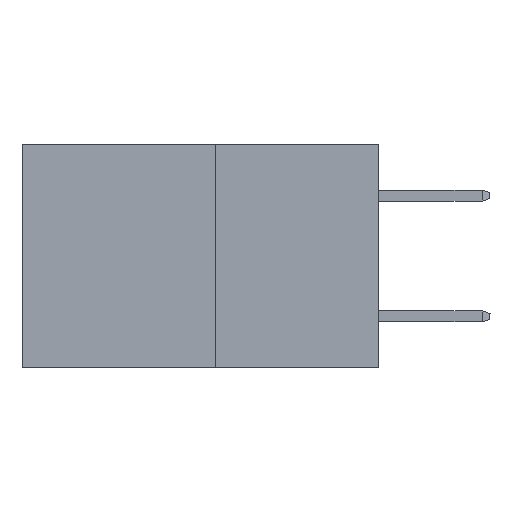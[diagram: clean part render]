
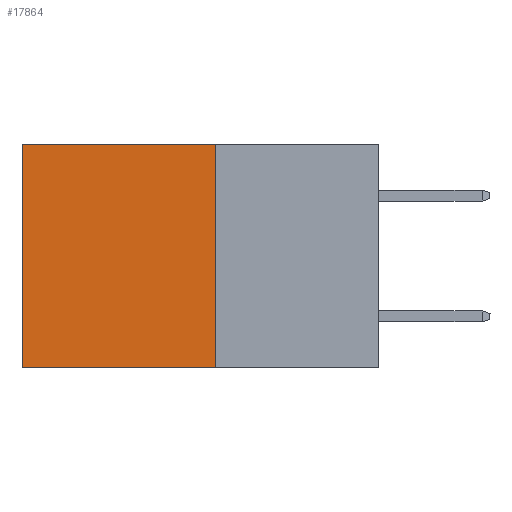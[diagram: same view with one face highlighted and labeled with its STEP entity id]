
A CAD part, left-side view. The second image highlights one B-rep face of the part: STEP entity #17864.
In plain terms, the highlighted planar face has unit normal (-1, 0, 0).
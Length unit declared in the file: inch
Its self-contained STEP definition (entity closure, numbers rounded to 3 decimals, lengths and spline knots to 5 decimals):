
#908 = EDGE_CURVE ( 'NONE', #5093, #25256, #27764, .T. ) ;
#1171 = EDGE_CURVE ( 'NONE', #25256, #20747, #2699, .T. ) ;
#1892 = CARTESIAN_POINT ( 'NONE',  ( 0.277, 0.27, 0. ) ) ;
#2695 = ORIENTED_EDGE ( 'NONE', *, *, #26985, .T. ) ;
#2699 = LINE ( 'NONE', #10954, #20624 ) ;
#3648 = FACE_OUTER_BOUND ( 'NONE', #4372, .T. ) ;
#4372 = EDGE_LOOP ( 'NONE', ( #29742, #8866, #21916, #2695 ) ) ;
#5093 = VERTEX_POINT ( 'NONE', #20848 ) ;
#6348 = LINE ( 'NONE', #1892, #24826 ) ;
#8408 = DIRECTION ( 'NONE',  ( 1., 0., 0. ) ) ;
#8866 = ORIENTED_EDGE ( 'NONE', *, *, #1171, .F. ) ;
#9906 = VERTEX_POINT ( 'NONE', #19849 ) ;
#10954 = CARTESIAN_POINT ( 'NONE',  ( 0.277, 0.27, -0.37 ) ) ;
#11597 = DIRECTION ( 'NONE',  ( 0., 0., -1. ) ) ;
#12564 = CARTESIAN_POINT ( 'NONE',  ( 0.277, 0.27, -0.37 ) ) ;
#12567 = DIRECTION ( 'NONE',  ( 0., 1., 0. ) ) ;
#14013 = AXIS2_PLACEMENT_3D ( 'NONE', #15394, #8408, #24552 ) ;
#15394 = CARTESIAN_POINT ( 'NONE',  ( 0.277, 0.27, -0.37 ) ) ;
#16998 = DIRECTION ( 'NONE',  ( 0., 0., -1. ) ) ;
#17706 = PLANE ( 'NONE',  #14013 ) ;
#17864 = ADVANCED_FACE ( 'NONE', ( #3648 ), #17706, .F. ) ;
#18308 = DIRECTION ( 'NONE',  ( 0., 1., 0. ) ) ;
#18896 = CARTESIAN_POINT ( 'NONE',  ( 0.277, 0.59, -0.37 ) ) ;
#19849 = CARTESIAN_POINT ( 'NONE',  ( 0.277, 0.59, 0. ) ) ;
#20624 = VECTOR ( 'NONE', #12567, 39.37008 ) ;
#20747 = VERTEX_POINT ( 'NONE', #18896 ) ;
#20848 = CARTESIAN_POINT ( 'NONE',  ( 0.277, 0.27, 0. ) ) ;
#21480 = VECTOR ( 'NONE', #11597, 39.37008 ) ;
#21916 = ORIENTED_EDGE ( 'NONE', *, *, #908, .F. ) ;
#22429 = VECTOR ( 'NONE', #16998, 39.37008 ) ;
#22473 = EDGE_CURVE ( 'NONE', #9906, #20747, #27510, .T. ) ;
#23272 = CARTESIAN_POINT ( 'NONE',  ( 0.277, 0.27, -0.37 ) ) ;
#24552 = DIRECTION ( 'NONE',  ( 0., 0., -1. ) ) ;
#24826 = VECTOR ( 'NONE', #18308, 39.37008 ) ;
#25256 = VERTEX_POINT ( 'NONE', #12564 ) ;
#25334 = CARTESIAN_POINT ( 'NONE',  ( 0.277, 0.59, -0.37 ) ) ;
#26985 = EDGE_CURVE ( 'NONE', #5093, #9906, #6348, .T. ) ;
#27510 = LINE ( 'NONE', #25334, #21480 ) ;
#27764 = LINE ( 'NONE', #23272, #22429 ) ;
#29742 = ORIENTED_EDGE ( 'NONE', *, *, #22473, .T. ) ;
